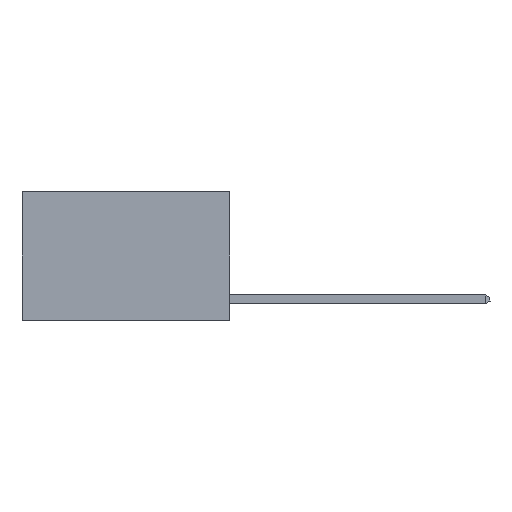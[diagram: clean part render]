
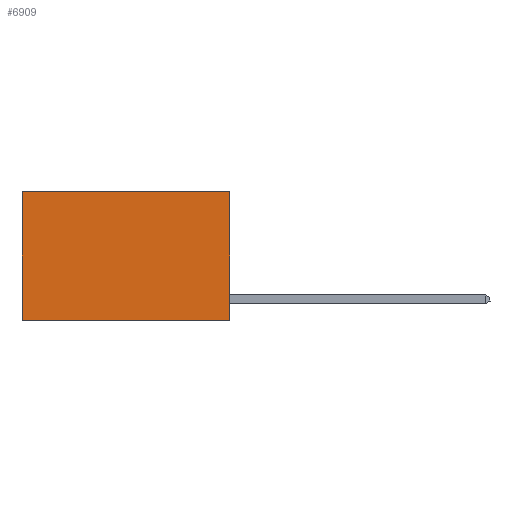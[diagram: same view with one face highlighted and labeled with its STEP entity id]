
A CAD part, left-side view. The second image highlights one B-rep face of the part: STEP entity #6909.
In plain terms, the highlighted planar face has unit normal (-1, 0, 0).
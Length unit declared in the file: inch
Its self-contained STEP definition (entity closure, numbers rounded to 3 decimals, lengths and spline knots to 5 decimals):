
#319 = VECTOR ( 'NONE', #11475, 39.37008 ) ;
#462 = EDGE_CURVE ( 'NONE', #10596, #5016, #4769, .T. ) ;
#737 = DIRECTION ( 'NONE',  ( 1., 0., 0. ) ) ;
#1342 = CARTESIAN_POINT ( 'NONE',  ( 0.2625, 0.6, -0.37 ) ) ;
#1576 = CARTESIAN_POINT ( 'NONE',  ( 0.2625, 0., 0. ) ) ;
#1617 = EDGE_LOOP ( 'NONE', ( #8916, #6542, #9720, #8529 ) ) ;
#1627 = CARTESIAN_POINT ( 'NONE',  ( 0.2625, 0., 0. ) ) ;
#2098 = CARTESIAN_POINT ( 'NONE',  ( 0.2625, 0., 0. ) ) ;
#2931 = AXIS2_PLACEMENT_3D ( 'NONE', #11520, #737, #6090 ) ;
#3164 = CARTESIAN_POINT ( 'NONE',  ( 0.2625, 0., -0.37 ) ) ;
#3169 = LINE ( 'NONE', #1576, #319 ) ;
#3614 = VECTOR ( 'NONE', #10280, 39.37008 ) ;
#3637 = DIRECTION ( 'NONE',  ( 0., 0., -1. ) ) ;
#4769 = LINE ( 'NONE', #2098, #10720 ) ;
#4857 = DIRECTION ( 'NONE',  ( 0., 1., 0. ) ) ;
#5016 = VERTEX_POINT ( 'NONE', #10425 ) ;
#5427 = FACE_OUTER_BOUND ( 'NONE', #1617, .T. ) ;
#5987 = EDGE_CURVE ( 'NONE', #10596, #8933, #3169, .T. ) ;
#6090 = DIRECTION ( 'NONE',  ( 0., 0., -1. ) ) ;
#6435 = EDGE_CURVE ( 'NONE', #8933, #10489, #10675, .T. ) ;
#6542 = ORIENTED_EDGE ( 'NONE', *, *, #6435, .F. ) ;
#6909 = ADVANCED_FACE ( 'NONE', ( #5427 ), #10634, .F. ) ;
#7248 = LINE ( 'NONE', #8064, #8811 ) ;
#7396 = EDGE_CURVE ( 'NONE', #5016, #10489, #7248, .T. ) ;
#8064 = CARTESIAN_POINT ( 'NONE',  ( 0.2625, 0.6, 0. ) ) ;
#8274 = CARTESIAN_POINT ( 'NONE',  ( 0.2625, 0., -0.37 ) ) ;
#8529 = ORIENTED_EDGE ( 'NONE', *, *, #462, .T. ) ;
#8811 = VECTOR ( 'NONE', #3637, 39.37008 ) ;
#8916 = ORIENTED_EDGE ( 'NONE', *, *, #7396, .T. ) ;
#8933 = VERTEX_POINT ( 'NONE', #8274 ) ;
#9720 = ORIENTED_EDGE ( 'NONE', *, *, #5987, .F. ) ;
#10280 = DIRECTION ( 'NONE',  ( 0., 1., 0. ) ) ;
#10425 = CARTESIAN_POINT ( 'NONE',  ( 0.2625, 0.6, 0. ) ) ;
#10489 = VERTEX_POINT ( 'NONE', #1342 ) ;
#10596 = VERTEX_POINT ( 'NONE', #1627 ) ;
#10634 = PLANE ( 'NONE',  #2931 ) ;
#10675 = LINE ( 'NONE', #3164, #3614 ) ;
#10720 = VECTOR ( 'NONE', #4857, 39.37008 ) ;
#11475 = DIRECTION ( 'NONE',  ( 0., 0., -1. ) ) ;
#11520 = CARTESIAN_POINT ( 'NONE',  ( 0.2625, 0., 0. ) ) ;
